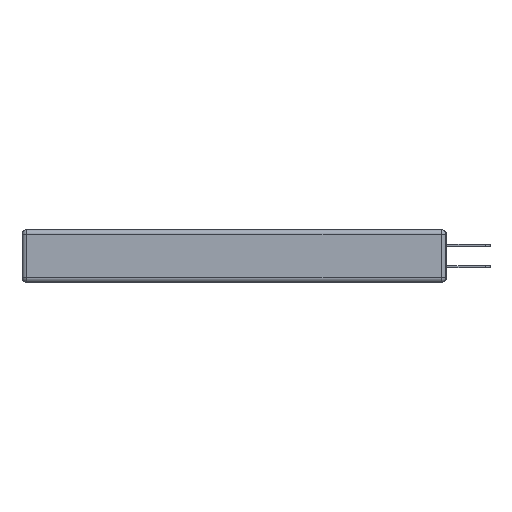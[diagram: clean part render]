
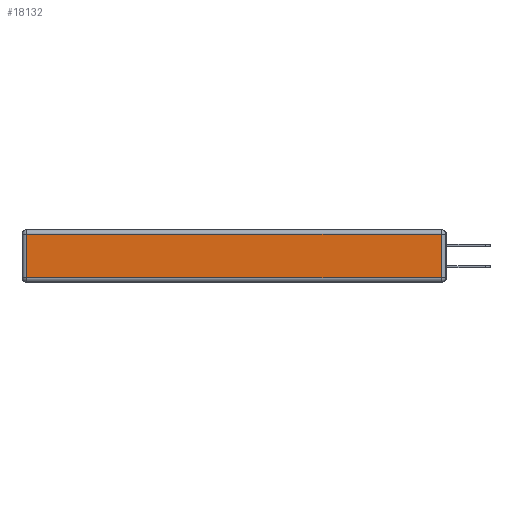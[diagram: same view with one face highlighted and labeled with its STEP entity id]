
A CAD part, left-side view. The second image highlights one B-rep face of the part: STEP entity #18132.
In plain terms, the highlighted planar face has unit normal (-1, 0, 0).
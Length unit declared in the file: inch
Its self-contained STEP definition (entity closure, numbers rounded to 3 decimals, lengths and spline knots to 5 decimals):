
#1446 = CARTESIAN_POINT ( 'NONE',  ( 0., 2.72, -0.03 ) ) ;
#1576 = FACE_OUTER_BOUND ( 'NONE', #21597, .T. ) ;
#1676 = EDGE_CURVE ( 'NONE', #7640, #23054, #14696, .T. ) ;
#1859 = CARTESIAN_POINT ( 'NONE',  ( 0., 0., -0.343 ) ) ;
#2836 = VECTOR ( 'NONE', #7227, 39.37008 ) ;
#4411 = ORIENTED_EDGE ( 'NONE', *, *, #1676, .T. ) ;
#4636 = EDGE_CURVE ( 'NONE', #23054, #10581, #20179, .T. ) ;
#6069 = LINE ( 'NONE', #20392, #9799 ) ;
#7179 = ORIENTED_EDGE ( 'NONE', *, *, #4636, .T. ) ;
#7227 = DIRECTION ( 'NONE',  ( 0., 0., -1. ) ) ;
#7640 = VERTEX_POINT ( 'NONE', #23306 ) ;
#7919 = ORIENTED_EDGE ( 'NONE', *, *, #17569, .T. ) ;
#8085 = CARTESIAN_POINT ( 'NONE',  ( 0., 0., -0.313 ) ) ;
#9799 = VECTOR ( 'NONE', #10350, 39.37008 ) ;
#10350 = DIRECTION ( 'NONE',  ( 0., 0., 1. ) ) ;
#10400 = CARTESIAN_POINT ( 'NONE',  ( 0., 2.72, -0.313 ) ) ;
#10581 = VERTEX_POINT ( 'NONE', #10400 ) ;
#13046 = LINE ( 'NONE', #8085, #23162 ) ;
#13174 = CARTESIAN_POINT ( 'NONE',  ( 0., 2.72, -0.343 ) ) ;
#13784 = ORIENTED_EDGE ( 'NONE', *, *, #22098, .T. ) ;
#14696 = LINE ( 'NONE', #19591, #24797 ) ;
#15793 = PLANE ( 'NONE',  #24576 ) ;
#17070 = VERTEX_POINT ( 'NONE', #24487 ) ;
#17569 = EDGE_CURVE ( 'NONE', #17070, #7640, #6069, .T. ) ;
#17811 = DIRECTION ( 'NONE',  ( -1., 0., 0. ) ) ;
#18132 = ADVANCED_FACE ( 'NONE', ( #1576 ), #15793, .T. ) ;
#19591 = CARTESIAN_POINT ( 'NONE',  ( 0., 2.75, -0.03 ) ) ;
#19837 = DIRECTION ( 'NONE',  ( 0., 0., 1. ) ) ;
#20179 = LINE ( 'NONE', #13174, #2836 ) ;
#20392 = CARTESIAN_POINT ( 'NONE',  ( 0., 0.03, -0.343 ) ) ;
#21597 = EDGE_LOOP ( 'NONE', ( #13784, #7919, #4411, #7179 ) ) ;
#21713 = DIRECTION ( 'NONE',  ( 0., 1., 0. ) ) ;
#22098 = EDGE_CURVE ( 'NONE', #10581, #17070, #13046, .T. ) ;
#23054 = VERTEX_POINT ( 'NONE', #1446 ) ;
#23162 = VECTOR ( 'NONE', #26109, 39.37008 ) ;
#23306 = CARTESIAN_POINT ( 'NONE',  ( 0., 0.03, -0.03 ) ) ;
#24487 = CARTESIAN_POINT ( 'NONE',  ( 0., 0.03, -0.313 ) ) ;
#24576 = AXIS2_PLACEMENT_3D ( 'NONE', #1859, #17811, #19837 ) ;
#24797 = VECTOR ( 'NONE', #21713, 39.37008 ) ;
#26109 = DIRECTION ( 'NONE',  ( 0., -1., 0. ) ) ;
